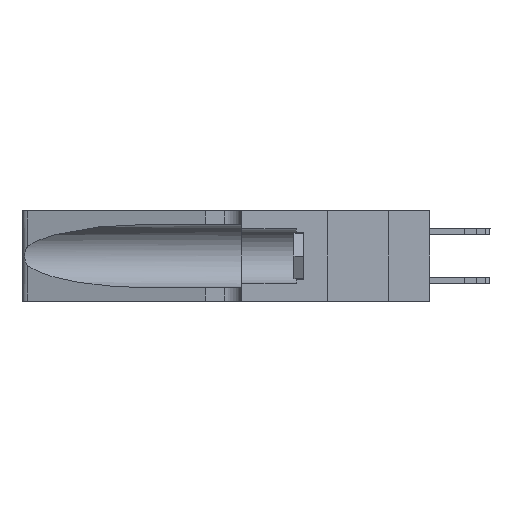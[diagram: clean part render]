
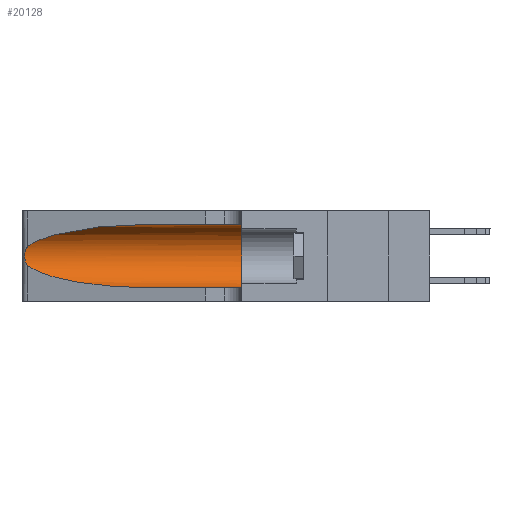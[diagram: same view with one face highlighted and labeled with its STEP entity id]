
A CAD part, left-side view. The second image highlights one B-rep face of the part: STEP entity #20128.
In plain terms, the highlighted cylindrical face has radius 3.308 mm (diameter 6.617 mm), a partial arc.
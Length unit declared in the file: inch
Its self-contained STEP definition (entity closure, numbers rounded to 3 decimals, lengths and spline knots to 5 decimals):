
#81 = ORIENTED_EDGE ( 'NONE', *, *, #9315, .T. ) ;
#207 = VERTEX_POINT ( 'NONE', #13921 ) ;
#569 = CARTESIAN_POINT ( 'NONE',  ( 0.25487, 1.22718, 0.14631 ) ) ;
#636 = CARTESIAN_POINT ( 'NONE',  ( 0.26017, 1.23833, 0.17102 ) ) ;
#1487 = ORIENTED_EDGE ( 'NONE', *, *, #4253, .T. ) ;
#1654 = EDGE_CURVE ( 'NONE', #3961, #3288, #17991, .T. ) ;
#2255 = VERTEX_POINT ( 'NONE', #12576 ) ;
#2290 = CARTESIAN_POINT ( 'NONE',  ( 0.25487, 1.22718, 0.22369 ) ) ;
#2693 = CARTESIAN_POINT ( 'NONE',  ( 0.1305, 1.61858, 0.185 ) ) ;
#2764 = EDGE_CURVE ( 'NONE', #3288, #11396, #4594, .T. ) ;
#2839 = DIRECTION ( 'NONE',  ( 0., -1., 0. ) ) ;
#3288 = VERTEX_POINT ( 'NONE', #10521 ) ;
#3472 = CARTESIAN_POINT ( 'NONE',  ( 0.1305, 1.61858, 0.05475 ) ) ;
#3685 = CARTESIAN_POINT ( 'NONE',  ( 0.1305, 0.35, 0.185 ) ) ;
#3961 = VERTEX_POINT ( 'NONE', #17029 ) ;
#4253 = EDGE_CURVE ( 'NONE', #207, #21214, #16990, .T. ) ;
#4594 = CIRCLE ( 'NONE', #8774, 0.13025 ) ;
#5506 = CARTESIAN_POINT ( 'NONE',  ( 0.25555, 1.22994, 0.2215 ) ) ;
#5617 = CYLINDRICAL_SURFACE ( 'NONE', #18762, 0.13025 ) ;
#5783 = CARTESIAN_POINT ( 'NONE',  ( 0.25487, 1.22718, 0.14631 ) ) ;
#5879 = ORIENTED_EDGE ( 'NONE', *, *, #2764, .F. ) ;
#6224 = VECTOR ( 'NONE', #15431, 39.37008 ) ;
#6408 = CARTESIAN_POINT ( 'NONE',  ( 0.1305, 0.72297, 0.05475 ) ) ;
#6613 = CARTESIAN_POINT ( 'NONE',  ( 0.2373, 1.15595, 0.08982 ) ) ;
#7520 = CARTESIAN_POINT ( 'NONE',  ( 0.26018, 1.23835, 0.19895 ) ) ;
#8219 = EDGE_CURVE ( 'NONE', #2255, #11396, #21779, .T. ) ;
#8499 = ORIENTED_EDGE ( 'NONE', *, *, #15459, .T. ) ;
#8774 = AXIS2_PLACEMENT_3D ( 'NONE', #3685, #19350, #8913 ) ;
#8913 = DIRECTION ( 'NONE',  ( 0., 0., 1. ) ) ;
#8941 = CARTESIAN_POINT ( 'NONE',  ( 0.25789, 1.23486, 0.15765 ) ) ;
#9102 = CARTESIAN_POINT ( 'NONE',  ( 0.25856, 1.23593, 0.16098 ) ) ;
#9315 = EDGE_CURVE ( 'NONE', #21214, #2255, #19918, .T. ) ;
#10263 = CARTESIAN_POINT ( 'NONE',  ( 0.2373, 1.15595, 0.28018 ) ) ;
#10521 = CARTESIAN_POINT ( 'NONE',  ( 0.1305, 0.35, 0.31525 ) ) ;
#10754 = CARTESIAN_POINT ( 'NONE',  ( 0.26075, 1.23896, 0.19203 ) ) ;
#10980 = CARTESIAN_POINT ( 'NONE',  ( 0.25787, 1.23484, 0.2124 ) ) ;
#11257 = FACE_OUTER_BOUND ( 'NONE', #12558, .T. ) ;
#11396 = VERTEX_POINT ( 'NONE', #21079 ) ;
#11605 = VECTOR ( 'NONE', #19041, 39.37008 ) ;
#12538 = CARTESIAN_POINT ( 'NONE',  ( 0.25555, 1.22993, 0.14849 ) ) ;
#12558 = EDGE_LOOP ( 'NONE', ( #8499, #1487, #81, #17114, #5879, #15385 ) ) ;
#12576 = CARTESIAN_POINT ( 'NONE',  ( 0.1305, 0.72297, 0.05475 ) ) ;
#13921 = CARTESIAN_POINT ( 'NONE',  ( 0.25487, 1.22718, 0.22369 ) ) ;
#14836 = CARTESIAN_POINT ( 'NONE',  ( 0.18966, 0.96281, 0.31525 ) ) ;
#15070 =( BOUNDED_CURVE ( )  B_SPLINE_CURVE ( 3, ( #18417, #14836, #10263, #21948 ),
 .UNSPECIFIED., .F., .F. ) 
 B_SPLINE_CURVE_WITH_KNOTS ( ( 4, 4 ),
 ( 1.5708, 2.84003 ),
 .UNSPECIFIED. ) 
 CURVE ( )  GEOMETRIC_REPRESENTATION_ITEM ( )  RATIONAL_B_SPLINE_CURVE ( ( 1., 0.87, 0.87, 1. ) ) 
 REPRESENTATION_ITEM ( '' )  );
#15097 = CARTESIAN_POINT ( 'NONE',  ( 0.18966, 0.96281, 0.05475 ) ) ;
#15385 = ORIENTED_EDGE ( 'NONE', *, *, #1654, .F. ) ;
#15431 = DIRECTION ( 'NONE',  ( 0., -1., 0. ) ) ;
#15459 = EDGE_CURVE ( 'NONE', #3961, #207, #15070, .T. ) ;
#16990 = B_SPLINE_CURVE_WITH_KNOTS ( 'NONE', 3,
 ( #2290, #5506, #17479, #10980, #17630, #7520, #10754, #19381, #636, #9102, #8941, #21094, #12538, #569 ),
 .UNSPECIFIED., .F., .F.,
 ( 4, 2, 2, 2, 2, 2, 4 ),
 ( 0., 0.00027, 0.00053, 0.00107, 0.0016, 0.00187, 0.00214 ),
 .UNSPECIFIED. ) ;
#17029 = CARTESIAN_POINT ( 'NONE',  ( 0.1305, 0.72297, 0.31525 ) ) ;
#17114 = ORIENTED_EDGE ( 'NONE', *, *, #8219, .T. ) ;
#17227 = CARTESIAN_POINT ( 'NONE',  ( 0.1305, 1.61858, 0.31525 ) ) ;
#17479 = CARTESIAN_POINT ( 'NONE',  ( 0.25639, 1.23184, 0.21858 ) ) ;
#17630 = CARTESIAN_POINT ( 'NONE',  ( 0.25854, 1.2359, 0.20912 ) ) ;
#17991 = LINE ( 'NONE', #17227, #11605 ) ;
#18100 = DIRECTION ( 'NONE',  ( 0., 0., -1. ) ) ;
#18330 = CARTESIAN_POINT ( 'NONE',  ( 0.25487, 1.22718, 0.14631 ) ) ;
#18417 = CARTESIAN_POINT ( 'NONE',  ( 0.1305, 0.72297, 0.31525 ) ) ;
#18762 = AXIS2_PLACEMENT_3D ( 'NONE', #2693, #2839, #18100 ) ;
#19041 = DIRECTION ( 'NONE',  ( 0., -1., 0. ) ) ;
#19350 = DIRECTION ( 'NONE',  ( 0., 1., 0. ) ) ;
#19381 = CARTESIAN_POINT ( 'NONE',  ( 0.26075, 1.23896, 0.178 ) ) ;
#19918 =( BOUNDED_CURVE ( )  B_SPLINE_CURVE ( 3, ( #18330, #6613, #15097, #6408 ),
 .UNSPECIFIED., .F., .F. ) 
 B_SPLINE_CURVE_WITH_KNOTS ( ( 4, 4 ),
 ( 3.44316, 4.71239 ),
 .UNSPECIFIED. ) 
 CURVE ( )  GEOMETRIC_REPRESENTATION_ITEM ( )  RATIONAL_B_SPLINE_CURVE ( ( 1., 0.87, 0.87, 1. ) ) 
 REPRESENTATION_ITEM ( '' )  );
#20128 = ADVANCED_FACE ( 'NONE', ( #11257 ), #5617, .F. ) ;
#21079 = CARTESIAN_POINT ( 'NONE',  ( 0.1305, 0.35, 0.05475 ) ) ;
#21094 = CARTESIAN_POINT ( 'NONE',  ( 0.25639, 1.23186, 0.15144 ) ) ;
#21214 = VERTEX_POINT ( 'NONE', #5783 ) ;
#21779 = LINE ( 'NONE', #3472, #6224 ) ;
#21948 = CARTESIAN_POINT ( 'NONE',  ( 0.25487, 1.22718, 0.22369 ) ) ;
